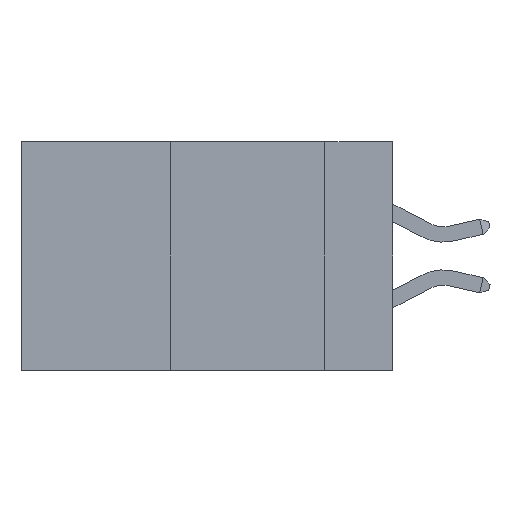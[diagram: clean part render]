
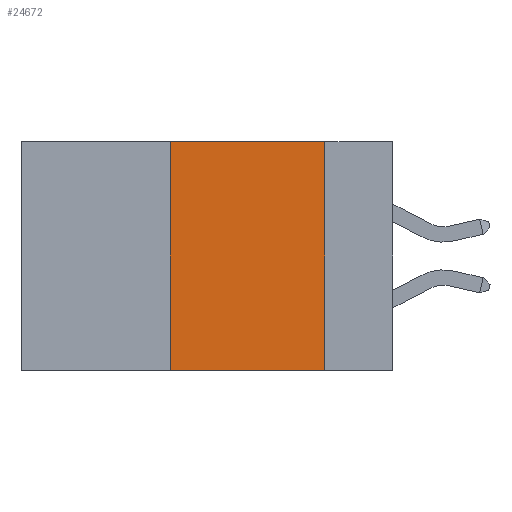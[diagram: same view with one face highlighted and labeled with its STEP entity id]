
A CAD part, left-side view. The second image highlights one B-rep face of the part: STEP entity #24672.
In plain terms, the highlighted planar face has unit normal (-1, 0, 0).
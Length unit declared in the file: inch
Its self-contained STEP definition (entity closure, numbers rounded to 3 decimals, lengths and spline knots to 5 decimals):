
#240 = VERTEX_POINT ( 'NONE', #5270 ) ;
#1204 = ORIENTED_EDGE ( 'NONE', *, *, #19903, .F. ) ;
#1328 = VECTOR ( 'NONE', #10456, 39.37008 ) ;
#2100 = PLANE ( 'NONE',  #20534 ) ;
#2252 = EDGE_CURVE ( 'NONE', #240, #22408, #17524, .T. ) ;
#2442 = VECTOR ( 'NONE', #28539, 39.37008 ) ;
#2708 = LINE ( 'NONE', #6122, #1328 ) ;
#4023 = VECTOR ( 'NONE', #14997, 39.37008 ) ;
#4863 = ORIENTED_EDGE ( 'NONE', *, *, #2252, .T. ) ;
#5038 = EDGE_CURVE ( 'NONE', #11907, #22408, #22930, .T. ) ;
#5270 = CARTESIAN_POINT ( 'NONE',  ( 0., 0.36, -0.37 ) ) ;
#5482 = FACE_OUTER_BOUND ( 'NONE', #21784, .T. ) ;
#5925 = LINE ( 'NONE', #7762, #24981 ) ;
#6122 = CARTESIAN_POINT ( 'NONE',  ( 0., 0.6, 0. ) ) ;
#7762 = CARTESIAN_POINT ( 'NONE',  ( 0., 0.36, 0. ) ) ;
#8466 = CARTESIAN_POINT ( 'NONE',  ( 0., 0.6, -0.37 ) ) ;
#8870 = DIRECTION ( 'NONE',  ( 1., 0., 0. ) ) ;
#10125 = ORIENTED_EDGE ( 'NONE', *, *, #22121, .F. ) ;
#10456 = DIRECTION ( 'NONE',  ( 0., -1., 0. ) ) ;
#11005 = CARTESIAN_POINT ( 'NONE',  ( 0., 0.11, 0. ) ) ;
#11895 = VERTEX_POINT ( 'NONE', #26129 ) ;
#11907 = VERTEX_POINT ( 'NONE', #11005 ) ;
#13963 = ORIENTED_EDGE ( 'NONE', *, *, #5038, .F. ) ;
#14997 = DIRECTION ( 'NONE',  ( 0., -1., 0. ) ) ;
#17425 = CARTESIAN_POINT ( 'NONE',  ( 0., 0.11, -0.37 ) ) ;
#17524 = LINE ( 'NONE', #8466, #4023 ) ;
#19838 = DIRECTION ( 'NONE',  ( 0., 0., -1. ) ) ;
#19903 = EDGE_CURVE ( 'NONE', #11895, #11907, #2708, .T. ) ;
#19929 = CARTESIAN_POINT ( 'NONE',  ( 0., 0.6, 0. ) ) ;
#20534 = AXIS2_PLACEMENT_3D ( 'NONE', #19929, #8870, #19838 ) ;
#21784 = EDGE_LOOP ( 'NONE', ( #13963, #1204, #10125, #4863 ) ) ;
#22121 = EDGE_CURVE ( 'NONE', #240, #11895, #5925, .T. ) ;
#22408 = VERTEX_POINT ( 'NONE', #17425 ) ;
#22930 = LINE ( 'NONE', #26529, #2442 ) ;
#24672 = ADVANCED_FACE ( 'NONE', ( #5482 ), #2100, .F. ) ;
#24981 = VECTOR ( 'NONE', #25623, 39.37008 ) ;
#25623 = DIRECTION ( 'NONE',  ( 0., 0., 1. ) ) ;
#26129 = CARTESIAN_POINT ( 'NONE',  ( 0., 0.36, 0. ) ) ;
#26529 = CARTESIAN_POINT ( 'NONE',  ( 0., 0.11, 0. ) ) ;
#28539 = DIRECTION ( 'NONE',  ( 0., 0., -1. ) ) ;
